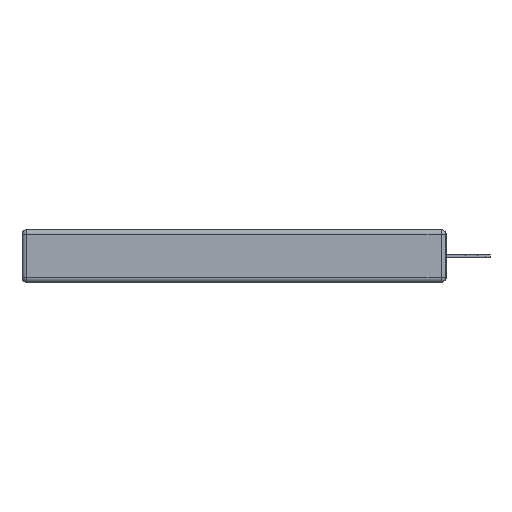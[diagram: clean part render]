
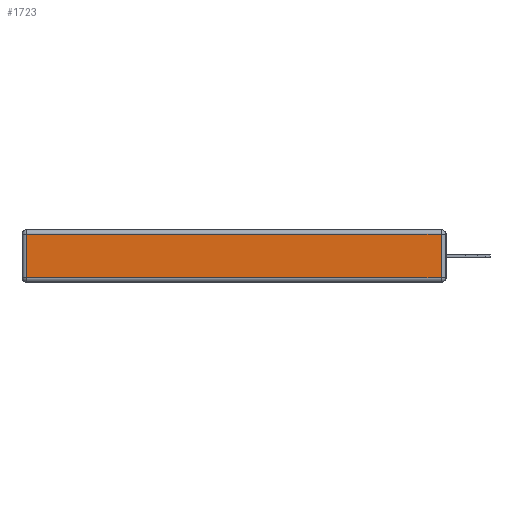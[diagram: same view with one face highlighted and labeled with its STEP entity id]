
A CAD part, left-side view. The second image highlights one B-rep face of the part: STEP entity #1723.
In plain terms, the highlighted planar face has unit normal (-1, 0, 0).
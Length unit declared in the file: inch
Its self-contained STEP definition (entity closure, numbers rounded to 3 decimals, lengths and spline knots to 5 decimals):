
#349 = ORIENTED_EDGE ( 'NONE', *, *, #24718, .T. ) ;
#453 = DIRECTION ( 'NONE',  ( 0., 0., 1. ) ) ;
#660 = FACE_OUTER_BOUND ( 'NONE', #24441, .T. ) ;
#800 = CARTESIAN_POINT ( 'NONE',  ( 0., 0., -0.343 ) ) ;
#1178 = ORIENTED_EDGE ( 'NONE', *, *, #28875, .T. ) ;
#1262 = ORIENTED_EDGE ( 'NONE', *, *, #23463, .T. ) ;
#1579 = CARTESIAN_POINT ( 'NONE',  ( 0., 2.72, -0.313 ) ) ;
#1595 = ORIENTED_EDGE ( 'NONE', *, *, #12302, .T. ) ;
#1723 = ADVANCED_FACE ( 'NONE', ( #660 ), #3041, .T. ) ;
#1782 = DIRECTION ( 'NONE',  ( 0., 1., 0. ) ) ;
#2737 = DIRECTION ( 'NONE',  ( -1., 0., 0. ) ) ;
#2876 = CARTESIAN_POINT ( 'NONE',  ( 0., 2.72, -0.03 ) ) ;
#3041 = PLANE ( 'NONE',  #16572 ) ;
#3920 = CARTESIAN_POINT ( 'NONE',  ( 0., 0.03, -0.03 ) ) ;
#3986 = VERTEX_POINT ( 'NONE', #2876 ) ;
#6101 = VERTEX_POINT ( 'NONE', #3920 ) ;
#6729 = LINE ( 'NONE', #22421, #26647 ) ;
#8005 = LINE ( 'NONE', #18283, #21863 ) ;
#9223 = VECTOR ( 'NONE', #15805, 39.37008 ) ;
#12302 = EDGE_CURVE ( 'NONE', #6101, #3986, #26397, .T. ) ;
#12404 = CARTESIAN_POINT ( 'NONE',  ( 0., 0.03, -0.313 ) ) ;
#13088 = VERTEX_POINT ( 'NONE', #1579 ) ;
#15805 = DIRECTION ( 'NONE',  ( 0., 0., -1. ) ) ;
#16572 = AXIS2_PLACEMENT_3D ( 'NONE', #800, #2737, #20830 ) ;
#17264 = CARTESIAN_POINT ( 'NONE',  ( 0., 2.75, -0.03 ) ) ;
#17752 = CARTESIAN_POINT ( 'NONE',  ( 0., 2.72, -0.343 ) ) ;
#18283 = CARTESIAN_POINT ( 'NONE',  ( 0., 0.03, -0.343 ) ) ;
#19889 = VECTOR ( 'NONE', #1782, 39.37008 ) ;
#20830 = DIRECTION ( 'NONE',  ( 0., 0., 1. ) ) ;
#21863 = VECTOR ( 'NONE', #453, 39.37008 ) ;
#22421 = CARTESIAN_POINT ( 'NONE',  ( 0., 0., -0.313 ) ) ;
#23463 = EDGE_CURVE ( 'NONE', #13088, #27347, #6729, .T. ) ;
#24441 = EDGE_LOOP ( 'NONE', ( #1262, #1178, #1595, #349 ) ) ;
#24513 = LINE ( 'NONE', #17752, #9223 ) ;
#24718 = EDGE_CURVE ( 'NONE', #3986, #13088, #24513, .T. ) ;
#25200 = DIRECTION ( 'NONE',  ( 0., -1., 0. ) ) ;
#26397 = LINE ( 'NONE', #17264, #19889 ) ;
#26647 = VECTOR ( 'NONE', #25200, 39.37008 ) ;
#27347 = VERTEX_POINT ( 'NONE', #12404 ) ;
#28875 = EDGE_CURVE ( 'NONE', #27347, #6101, #8005, .T. ) ;
